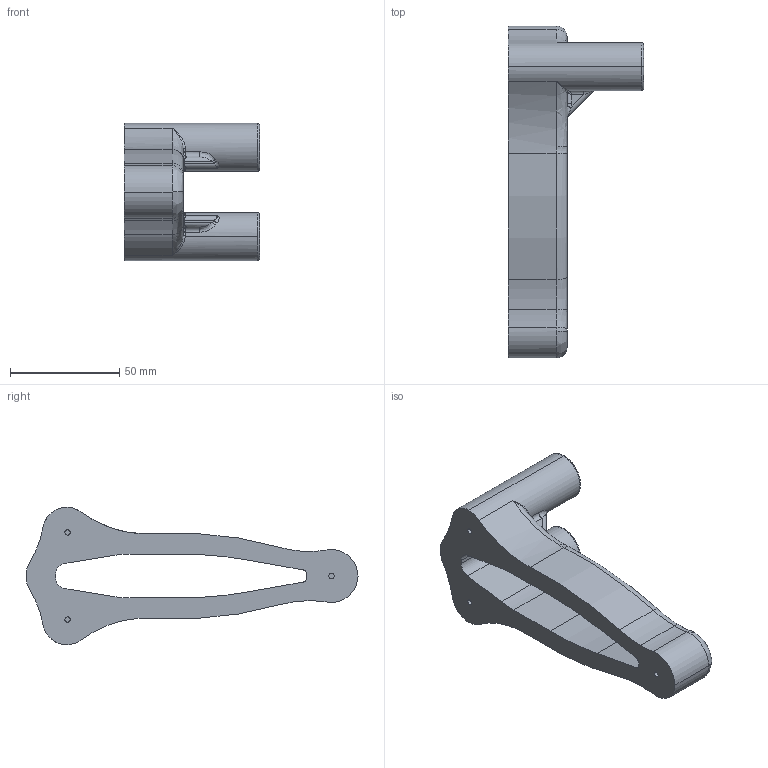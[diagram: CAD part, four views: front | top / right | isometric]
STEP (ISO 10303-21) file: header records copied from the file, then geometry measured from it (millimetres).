
FILE_DESCRIPTION (( 'STEP AP203' ), '1' );
FILE_NAME ('BUTT STOCK.STEP', '2020-09-28T01:15:08', ( '' ), ( '' ), 'SwSTEP 2.0', 'SolidWorks 2019', '' );
FILE_SCHEMA (( 'CONFIG_CONTROL_DESIGN' ));
Length unit declared in the file: millimetre
Products named in the file (1): BUTT STOCK
Bounding box: 62 x 152.22 x 63 mm (x, y, z)
Volume: 124556.9 mm3; surface area: 29806.5 mm2
Topology: 1 solids, 1 shells, 152 faces, 370 edges, 216 vertices
Faces by surface type: bspline 64, cylinder 59, plane 27, torus 2
Entity records: 6396 total; most frequent: CARTESIAN_POINT 3251, ORIENTED_EDGE 724, DIRECTION 528, EDGE_CURVE 362, VERTEX_POINT 216, AXIS2_PLACEMENT_3D 212, EDGE_LOOP 158, FACE_OUTER_BOUND 152
